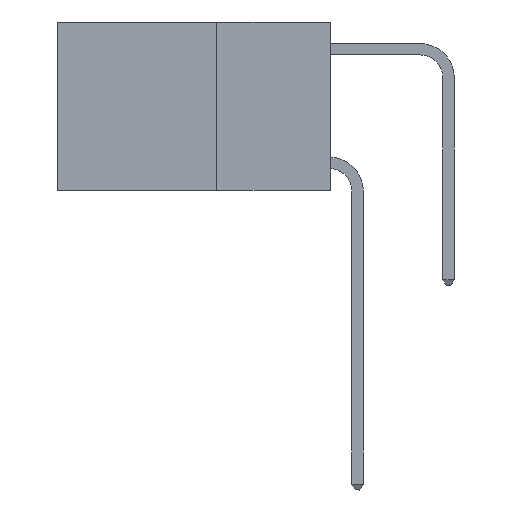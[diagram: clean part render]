
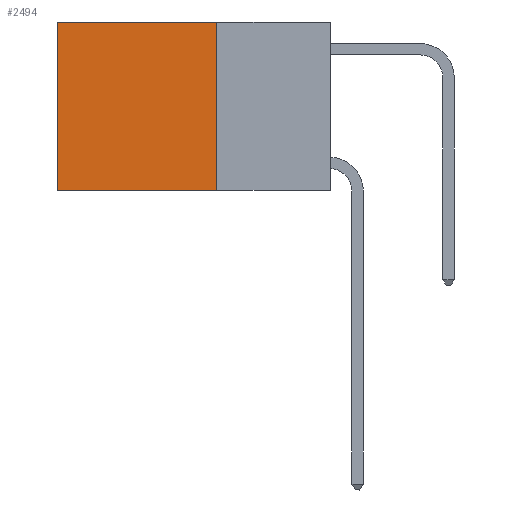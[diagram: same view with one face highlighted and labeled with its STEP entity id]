
A CAD part, left-side view. The second image highlights one B-rep face of the part: STEP entity #2494.
In plain terms, the highlighted planar face has unit normal (-1, 0, 0).
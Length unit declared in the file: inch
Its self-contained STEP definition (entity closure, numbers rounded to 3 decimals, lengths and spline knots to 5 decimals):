
#384 = EDGE_CURVE ( 'NONE', #18367, #16237, #6153, .T. ) ;
#549 = EDGE_CURVE ( 'NONE', #9864, #16185, #15534, .T. ) ;
#1061 = EDGE_CURVE ( 'NONE', #16185, #16237, #15027, .T. ) ;
#2296 = EDGE_CURVE ( 'NONE', #9864, #18367, #8409, .T. ) ;
#2494 = ADVANCED_FACE ( 'NONE', ( #10945 ), #5463, .F. ) ;
#5463 = PLANE ( 'NONE',  #20593 ) ;
#5547 = CARTESIAN_POINT ( 'NONE',  ( 0.2625, 0.25, -0.37 ) ) ;
#5889 = ORIENTED_EDGE ( 'NONE', *, *, #384, .F. ) ;
#6153 = LINE ( 'NONE', #7309, #14318 ) ;
#6624 = ORIENTED_EDGE ( 'NONE', *, *, #549, .T. ) ;
#7109 = ORIENTED_EDGE ( 'NONE', *, *, #2296, .F. ) ;
#7166 = DIRECTION ( 'NONE',  ( 0., 0., -1. ) ) ;
#7274 = CARTESIAN_POINT ( 'NONE',  ( 0.2625, 0.6, 0. ) ) ;
#7309 = CARTESIAN_POINT ( 'NONE',  ( 0.2625, 0.25, -0.37 ) ) ;
#7834 = DIRECTION ( 'NONE',  ( 0., 0., -1. ) ) ;
#8409 = LINE ( 'NONE', #20422, #12210 ) ;
#9086 = DIRECTION ( 'NONE',  ( 0., 1., 0. ) ) ;
#9605 = DIRECTION ( 'NONE',  ( 0., 0., -1. ) ) ;
#9864 = VERTEX_POINT ( 'NONE', #19581 ) ;
#10717 = EDGE_LOOP ( 'NONE', ( #19461, #5889, #7109, #6624 ) ) ;
#10763 = VECTOR ( 'NONE', #9605, 39.37008 ) ;
#10945 = FACE_OUTER_BOUND ( 'NONE', #10717, .T. ) ;
#12210 = VECTOR ( 'NONE', #7834, 39.37008 ) ;
#12285 = VECTOR ( 'NONE', #9086, 39.37008 ) ;
#14318 = VECTOR ( 'NONE', #17603, 39.37008 ) ;
#14631 = CARTESIAN_POINT ( 'NONE',  ( 0.2625, 0.25, 0. ) ) ;
#15027 = LINE ( 'NONE', #7274, #10763 ) ;
#15534 = LINE ( 'NONE', #14631, #12285 ) ;
#16185 = VERTEX_POINT ( 'NONE', #20498 ) ;
#16237 = VERTEX_POINT ( 'NONE', #17629 ) ;
#16747 = DIRECTION ( 'NONE',  ( 1., 0., 0. ) ) ;
#17603 = DIRECTION ( 'NONE',  ( 0., 1., 0. ) ) ;
#17629 = CARTESIAN_POINT ( 'NONE',  ( 0.2625, 0.6, -0.37 ) ) ;
#18213 = CARTESIAN_POINT ( 'NONE',  ( 0.2625, 0.25, 0. ) ) ;
#18367 = VERTEX_POINT ( 'NONE', #5547 ) ;
#19461 = ORIENTED_EDGE ( 'NONE', *, *, #1061, .T. ) ;
#19581 = CARTESIAN_POINT ( 'NONE',  ( 0.2625, 0.25, 0. ) ) ;
#20422 = CARTESIAN_POINT ( 'NONE',  ( 0.2625, 0.25, 0. ) ) ;
#20498 = CARTESIAN_POINT ( 'NONE',  ( 0.2625, 0.6, 0. ) ) ;
#20593 = AXIS2_PLACEMENT_3D ( 'NONE', #18213, #16747, #7166 ) ;
